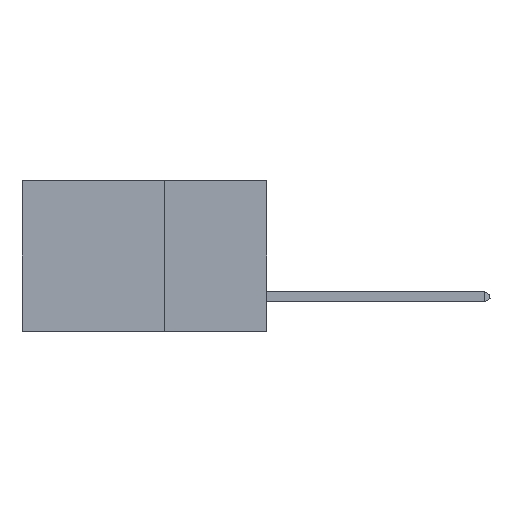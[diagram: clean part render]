
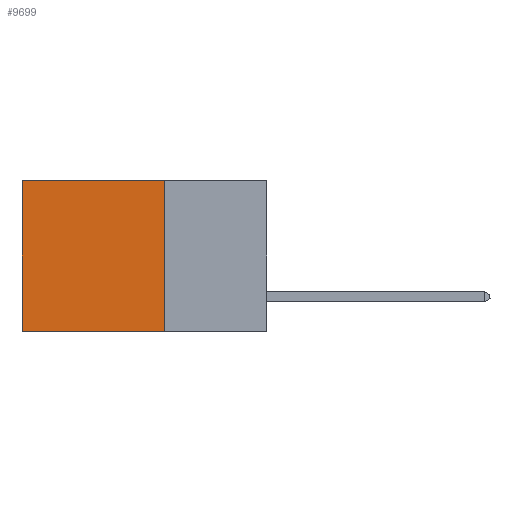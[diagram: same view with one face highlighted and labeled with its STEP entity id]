
A CAD part, left-side view. The second image highlights one B-rep face of the part: STEP entity #9699.
In plain terms, the highlighted planar face has unit normal (-1, 0, 0).
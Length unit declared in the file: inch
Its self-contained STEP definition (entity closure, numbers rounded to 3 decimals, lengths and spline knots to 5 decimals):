
#19 = LINE ( 'NONE', #21179, #21926 ) ;
#44 = DIRECTION ( 'NONE',  ( 0., 0., -1. ) ) ;
#716 = CARTESIAN_POINT ( 'NONE',  ( 0.2875, 0.6, 0. ) ) ;
#1698 = DIRECTION ( 'NONE',  ( 0., 1., 0. ) ) ;
#3458 = LINE ( 'NONE', #4683, #18081 ) ;
#4522 = CARTESIAN_POINT ( 'NONE',  ( 0.2875, 0.25, 0. ) ) ;
#4683 = CARTESIAN_POINT ( 'NONE',  ( 0.2875, 0.25, -0.37 ) ) ;
#4739 = FACE_OUTER_BOUND ( 'NONE', #12374, .T. ) ;
#4817 = EDGE_CURVE ( 'NONE', #16466, #22438, #3458, .T. ) ;
#6231 = LINE ( 'NONE', #13849, #31390 ) ;
#7689 = ORIENTED_EDGE ( 'NONE', *, *, #4817, .F. ) ;
#8680 = ORIENTED_EDGE ( 'NONE', *, *, #31354, .F. ) ;
#9532 = CARTESIAN_POINT ( 'NONE',  ( 0.2875, 0.25, 0. ) ) ;
#9699 = ADVANCED_FACE ( 'NONE', ( #4739 ), #27956, .F. ) ;
#10464 = ORIENTED_EDGE ( 'NONE', *, *, #29260, .T. ) ;
#11583 = EDGE_CURVE ( 'NONE', #33529, #33394, #19, .T. ) ;
#12374 = EDGE_LOOP ( 'NONE', ( #10464, #7689, #8680, #36728 ) ) ;
#13095 = CARTESIAN_POINT ( 'NONE',  ( 0.2875, 0.6, -0.37 ) ) ;
#13632 = VECTOR ( 'NONE', #20705, 39.37008 ) ;
#13849 = CARTESIAN_POINT ( 'NONE',  ( 0.2875, 0.25, 0. ) ) ;
#15079 = DIRECTION ( 'NONE',  ( 0., 1., 0. ) ) ;
#16466 = VERTEX_POINT ( 'NONE', #20818 ) ;
#16488 = AXIS2_PLACEMENT_3D ( 'NONE', #4522, #25536, #44 ) ;
#18081 = VECTOR ( 'NONE', #1698, 39.37008 ) ;
#20705 = DIRECTION ( 'NONE',  ( 0., 0., -1. ) ) ;
#20818 = CARTESIAN_POINT ( 'NONE',  ( 0.2875, 0.25, -0.37 ) ) ;
#21179 = CARTESIAN_POINT ( 'NONE',  ( 0.2875, 0.25, 0. ) ) ;
#21294 = LINE ( 'NONE', #716, #13632 ) ;
#21926 = VECTOR ( 'NONE', #15079, 39.37008 ) ;
#22438 = VERTEX_POINT ( 'NONE', #13095 ) ;
#22632 = DIRECTION ( 'NONE',  ( 0., 0., -1. ) ) ;
#25536 = DIRECTION ( 'NONE',  ( 1., 0., 0. ) ) ;
#27956 = PLANE ( 'NONE',  #16488 ) ;
#29260 = EDGE_CURVE ( 'NONE', #33394, #22438, #21294, .T. ) ;
#31354 = EDGE_CURVE ( 'NONE', #33529, #16466, #6231, .T. ) ;
#31390 = VECTOR ( 'NONE', #22632, 39.37008 ) ;
#33394 = VERTEX_POINT ( 'NONE', #36741 ) ;
#33529 = VERTEX_POINT ( 'NONE', #9532 ) ;
#36728 = ORIENTED_EDGE ( 'NONE', *, *, #11583, .T. ) ;
#36741 = CARTESIAN_POINT ( 'NONE',  ( 0.2875, 0.6, 0. ) ) ;
